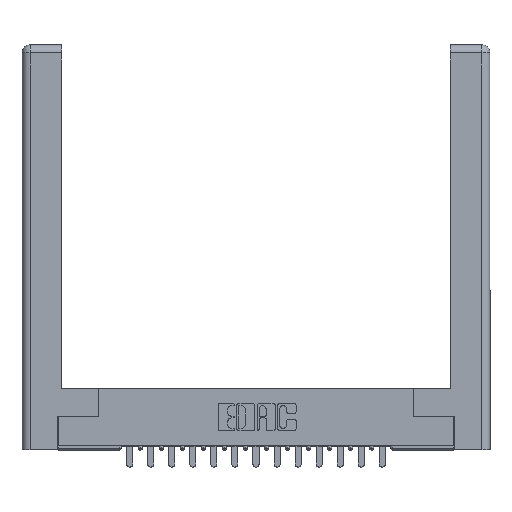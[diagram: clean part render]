
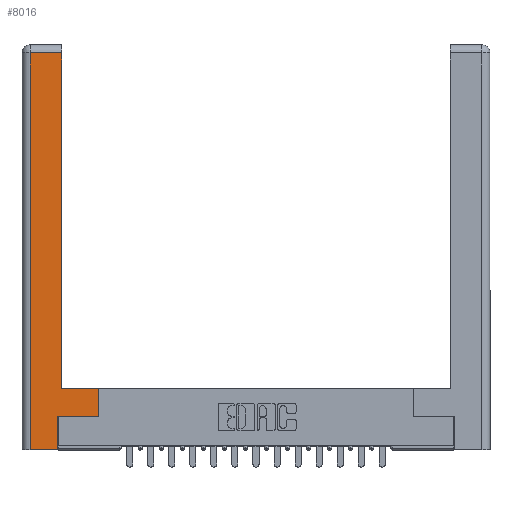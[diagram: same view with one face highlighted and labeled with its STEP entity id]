
A CAD part, top view. The second image highlights one B-rep face of the part: STEP entity #8016.
In plain terms, the highlighted planar face has unit normal (0, 0, 1).
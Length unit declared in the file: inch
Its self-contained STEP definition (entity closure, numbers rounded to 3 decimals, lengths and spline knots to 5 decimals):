
#98 = DIRECTION ( 'NONE',  ( 0., 1., 0. ) ) ;
#248 = CARTESIAN_POINT ( 'NONE',  ( 0.0615, 0., 0. ) ) ;
#331 = EDGE_CURVE ( 'NONE', #9009, #10375, #19814, .T. ) ;
#340 = LINE ( 'NONE', #5281, #18793 ) ;
#453 = CARTESIAN_POINT ( 'NONE',  ( 0.295, 0.45, 0. ) ) ;
#484 = ORIENTED_EDGE ( 'NONE', *, *, #9033, .T. ) ;
#742 = EDGE_CURVE ( 'NONE', #14526, #5862, #4030, .T. ) ;
#1403 = CARTESIAN_POINT ( 'NONE',  ( 0.0615, 0., 0. ) ) ;
#1752 = PLANE ( 'NONE',  #17718 ) ;
#1780 = DIRECTION ( 'NONE',  ( 1., 0., 0. ) ) ;
#2053 = DIRECTION ( 'NONE',  ( -1., 0., 0. ) ) ;
#2183 = EDGE_CURVE ( 'NONE', #10077, #9009, #13482, .T. ) ;
#2441 = CARTESIAN_POINT ( 'NONE',  ( 0.295, 2.94, 0. ) ) ;
#2708 = ORIENTED_EDGE ( 'NONE', *, *, #742, .T. ) ;
#2743 = ORIENTED_EDGE ( 'NONE', *, *, #331, .T. ) ;
#3269 = VERTEX_POINT ( 'NONE', #4199 ) ;
#3316 = DIRECTION ( 'NONE',  ( -1., 0., 0. ) ) ;
#3520 = LINE ( 'NONE', #11078, #18103 ) ;
#3644 = CARTESIAN_POINT ( 'NONE',  ( 0.565, 0.45, 0. ) ) ;
#3924 = CARTESIAN_POINT ( 'NONE',  ( 0.565, 0.45, 0. ) ) ;
#4030 = LINE ( 'NONE', #3924, #14502 ) ;
#4199 = CARTESIAN_POINT ( 'NONE',  ( 0.265, 0.245, 0. ) ) ;
#4301 = CARTESIAN_POINT ( 'NONE',  ( 0.295, 0.45, 0. ) ) ;
#4924 = VERTEX_POINT ( 'NONE', #14914 ) ;
#5095 = DIRECTION ( 'NONE',  ( 0., 0., -1. ) ) ;
#5281 = CARTESIAN_POINT ( 'NONE',  ( 0.265, 0.245, 0. ) ) ;
#5546 = CARTESIAN_POINT ( 'NONE',  ( 0.565, 0.245, 0. ) ) ;
#5862 = VERTEX_POINT ( 'NONE', #3644 ) ;
#6205 = ORIENTED_EDGE ( 'NONE', *, *, #8375, .T. ) ;
#6966 = VECTOR ( 'NONE', #18325, 39.37008 ) ;
#8016 = ADVANCED_FACE ( 'NONE', ( #11672 ), #1752, .F. ) ;
#8211 = CARTESIAN_POINT ( 'NONE',  ( 0.0615, 2.94, 0. ) ) ;
#8375 = EDGE_CURVE ( 'NONE', #5862, #16229, #18677, .T. ) ;
#8388 = ORIENTED_EDGE ( 'NONE', *, *, #2183, .T. ) ;
#9009 = VERTEX_POINT ( 'NONE', #8211 ) ;
#9033 = EDGE_CURVE ( 'NONE', #3269, #14526, #3520, .T. ) ;
#9282 = DIRECTION ( 'NONE',  ( 1., 0., 0. ) ) ;
#10077 = VERTEX_POINT ( 'NONE', #2441 ) ;
#10375 = VERTEX_POINT ( 'NONE', #248 ) ;
#10480 = VECTOR ( 'NONE', #9282, 39.37008 ) ;
#11078 = CARTESIAN_POINT ( 'NONE',  ( 0.565, 0.245, 0. ) ) ;
#11564 = CARTESIAN_POINT ( 'NONE',  ( 0.0615, 2.94, 0. ) ) ;
#11672 = FACE_OUTER_BOUND ( 'NONE', #14436, .T. ) ;
#11794 = CARTESIAN_POINT ( 'NONE',  ( 0.295, 3., 0. ) ) ;
#12111 = EDGE_CURVE ( 'NONE', #4924, #3269, #340, .T. ) ;
#13482 = LINE ( 'NONE', #11564, #14449 ) ;
#14132 = ORIENTED_EDGE ( 'NONE', *, *, #12111, .T. ) ;
#14358 = ORIENTED_EDGE ( 'NONE', *, *, #18576, .T. ) ;
#14436 = EDGE_LOOP ( 'NONE', ( #18125, #8388, #2743, #14358, #14132, #484, #2708, #6205 ) ) ;
#14449 = VECTOR ( 'NONE', #2053, 39.37008 ) ;
#14502 = VECTOR ( 'NONE', #14805, 39.37008 ) ;
#14526 = VERTEX_POINT ( 'NONE', #5546 ) ;
#14593 = VECTOR ( 'NONE', #16794, 39.37008 ) ;
#14805 = DIRECTION ( 'NONE',  ( 0., 1., 0. ) ) ;
#14841 = VECTOR ( 'NONE', #14925, 39.37008 ) ;
#14914 = CARTESIAN_POINT ( 'NONE',  ( 0.265, 0., 0. ) ) ;
#14925 = DIRECTION ( 'NONE',  ( 0., 1., 0. ) ) ;
#15835 = CARTESIAN_POINT ( 'NONE',  ( 0., 0., 0. ) ) ;
#16229 = VERTEX_POINT ( 'NONE', #453 ) ;
#16794 = DIRECTION ( 'NONE',  ( -1., 0., 0. ) ) ;
#17718 = AXIS2_PLACEMENT_3D ( 'NONE', #15835, #5095, #3316 ) ;
#18103 = VECTOR ( 'NONE', #1780, 39.37008 ) ;
#18125 = ORIENTED_EDGE ( 'NONE', *, *, #18250, .T. ) ;
#18250 = EDGE_CURVE ( 'NONE', #16229, #10077, #19447, .T. ) ;
#18325 = DIRECTION ( 'NONE',  ( 0., -1., 0. ) ) ;
#18543 = CARTESIAN_POINT ( 'NONE',  ( 0.265, 0., 0. ) ) ;
#18576 = EDGE_CURVE ( 'NONE', #10375, #4924, #18712, .T. ) ;
#18677 = LINE ( 'NONE', #4301, #14593 ) ;
#18712 = LINE ( 'NONE', #18543, #10480 ) ;
#18793 = VECTOR ( 'NONE', #98, 39.37008 ) ;
#19447 = LINE ( 'NONE', #11794, #14841 ) ;
#19814 = LINE ( 'NONE', #1403, #6966 ) ;
